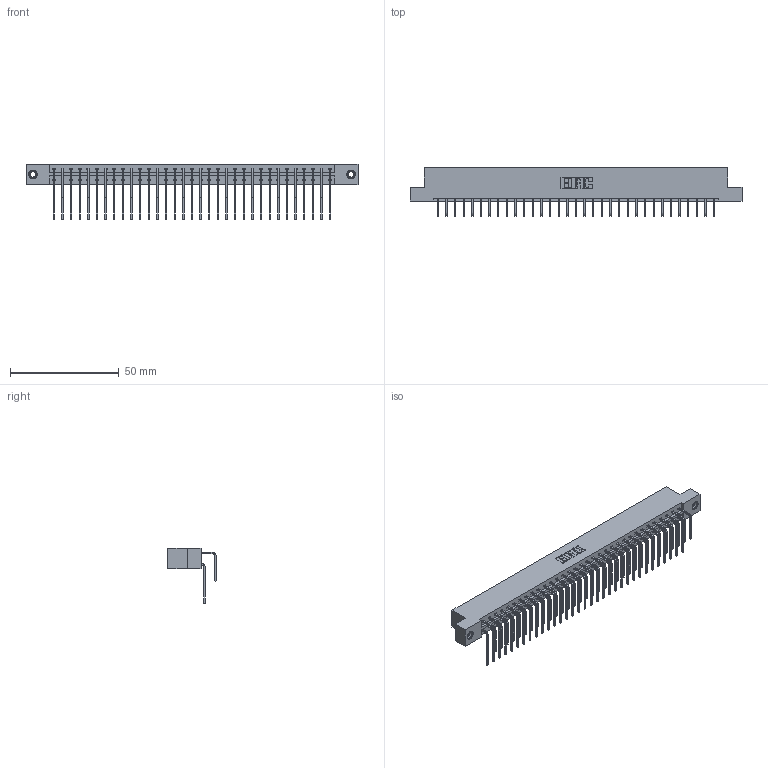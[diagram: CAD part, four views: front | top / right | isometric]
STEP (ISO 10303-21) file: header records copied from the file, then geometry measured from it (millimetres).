
FILE_DESCRIPTION (( 'STEP AP203' ), '1' );
FILE_NAME ('333-066-558-207.STEP', '2018-08-04T12:01:08', ( '' ), ( '' ), 'SwSTEP 2.0', 'SolidWorks 2016', '' );
FILE_SCHEMA (( 'CONFIG_CONTROL_DESIGN' ));
Length unit declared in the file: inch
Products named in the file (5): 345-250-001_345-250-005-103; 333-066-558-207; 333 Part_Flush - .156 Dia - TI; 345-292-001_558 559 Tail - 1; 345-292-001_558 Tail - 2
Assembly tree (69 placements, depth 2):
  333-066-558-207
    333 Part_Flush - .156 Dia - TI
    345-292-001_558 559 Tail - 1  x33
    345-292-001_558 Tail - 2  x33
    345-250-001_345-250-005-103  x2
Bounding box: 152.3 x 22.17 x 25.53 mm (x, y, z)
Volume: 15831.9 mm3; surface area: 20551.1 mm2
Topology: 69 solids, 69 shells, 3738 faces, 11073 edges, 7286 vertices
Faces by surface type: plane 2610, cylinder 1112, cone 12, torus 4
Entity records: 25364 total; most frequent: CARTESIAN_POINT 4248, ORIENTED_EDGE 4126, DIRECTION 3657, EDGE_CURVE 2063, LINE 1875, VECTOR 1875, VERTEX_POINT 1368, AXIS2_PLACEMENT_3D 891
